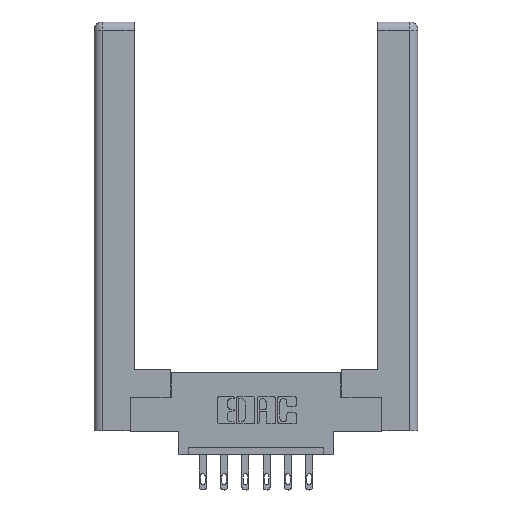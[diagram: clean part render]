
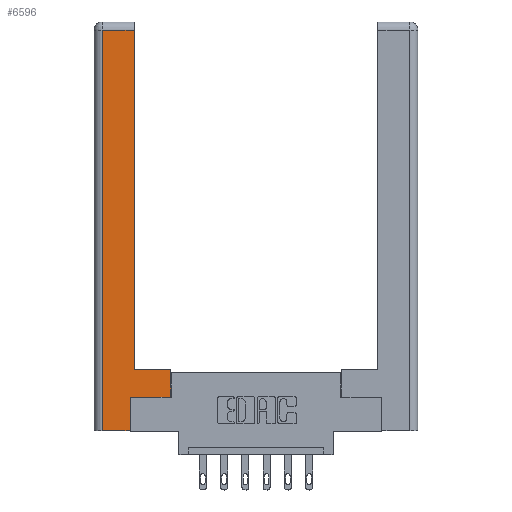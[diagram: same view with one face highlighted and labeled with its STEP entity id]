
A CAD part, top view. The second image highlights one B-rep face of the part: STEP entity #6596.
In plain terms, the highlighted planar face has unit normal (0, 0, 1).
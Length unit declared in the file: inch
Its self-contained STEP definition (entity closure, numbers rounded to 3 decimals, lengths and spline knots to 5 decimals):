
#57 = AXIS2_PLACEMENT_3D ( 'NONE', #5705, #9195, #6547 ) ;
#87 = CARTESIAN_POINT ( 'NONE',  ( 0.565, 0.45, 0. ) ) ;
#182 = LINE ( 'NONE', #9821, #8907 ) ;
#188 = DIRECTION ( 'NONE',  ( -1., 0., 0. ) ) ;
#192 = CARTESIAN_POINT ( 'NONE',  ( 0.0615, 0., 0. ) ) ;
#220 = DIRECTION ( 'NONE',  ( 0., 1., 0. ) ) ;
#345 = LINE ( 'NONE', #87, #2382 ) ;
#414 = FACE_OUTER_BOUND ( 'NONE', #2441, .T. ) ;
#625 = CARTESIAN_POINT ( 'NONE',  ( 0.295, 3., 0. ) ) ;
#692 = CARTESIAN_POINT ( 'NONE',  ( 0.0615, 2.94, 0. ) ) ;
#757 = CARTESIAN_POINT ( 'NONE',  ( 0.565, 0.45, 0. ) ) ;
#875 = LINE ( 'NONE', #4035, #4352 ) ;
#1170 = DIRECTION ( 'NONE',  ( 0., -1., 0. ) ) ;
#1419 = DIRECTION ( 'NONE',  ( 1., 0., 0. ) ) ;
#1443 = ORIENTED_EDGE ( 'NONE', *, *, #10647, .T. ) ;
#1577 = CARTESIAN_POINT ( 'NONE',  ( 0.265, 0., 0. ) ) ;
#1933 = ORIENTED_EDGE ( 'NONE', *, *, #9847, .T. ) ;
#2232 = VERTEX_POINT ( 'NONE', #1577 ) ;
#2312 = VERTEX_POINT ( 'NONE', #3712 ) ;
#2349 = CARTESIAN_POINT ( 'NONE',  ( 0.265, 0., 0. ) ) ;
#2382 = VECTOR ( 'NONE', #9279, 39.37008 ) ;
#2406 = ORIENTED_EDGE ( 'NONE', *, *, #5394, .T. ) ;
#2441 = EDGE_LOOP ( 'NONE', ( #3997, #5386, #6821, #2406, #8994, #1933, #6536, #1443 ) ) ;
#2784 = CARTESIAN_POINT ( 'NONE',  ( 0.0615, 0., 0. ) ) ;
#3058 = CARTESIAN_POINT ( 'NONE',  ( 0.295, 2.94, 0. ) ) ;
#3161 = EDGE_CURVE ( 'NONE', #2232, #4974, #3533, .T. ) ;
#3224 = VECTOR ( 'NONE', #9689, 39.37008 ) ;
#3470 = CARTESIAN_POINT ( 'NONE',  ( 0.565, 0.245, 0. ) ) ;
#3533 = LINE ( 'NONE', #6516, #9056 ) ;
#3712 = CARTESIAN_POINT ( 'NONE',  ( 0.295, 0.45, 0. ) ) ;
#3997 = ORIENTED_EDGE ( 'NONE', *, *, #7509, .T. ) ;
#4012 = EDGE_CURVE ( 'NONE', #9535, #5421, #4650, .T. ) ;
#4035 = CARTESIAN_POINT ( 'NONE',  ( 0.295, 0.45, 0. ) ) ;
#4266 = DIRECTION ( 'NONE',  ( 0., 1., 0. ) ) ;
#4352 = VECTOR ( 'NONE', #188, 39.37008 ) ;
#4417 = LINE ( 'NONE', #192, #9095 ) ;
#4650 = LINE ( 'NONE', #692, #3224 ) ;
#4974 = VERTEX_POINT ( 'NONE', #7138 ) ;
#5315 = DIRECTION ( 'NONE',  ( 1., 0., 0. ) ) ;
#5386 = ORIENTED_EDGE ( 'NONE', *, *, #4012, .T. ) ;
#5394 = EDGE_CURVE ( 'NONE', #10939, #2232, #9746, .T. ) ;
#5421 = VERTEX_POINT ( 'NONE', #10515 ) ;
#5469 = VECTOR ( 'NONE', #1419, 39.37008 ) ;
#5705 = CARTESIAN_POINT ( 'NONE',  ( 0., 0., 0. ) ) ;
#5869 = VERTEX_POINT ( 'NONE', #3470 ) ;
#6516 = CARTESIAN_POINT ( 'NONE',  ( 0.265, 0.245, 0. ) ) ;
#6536 = ORIENTED_EDGE ( 'NONE', *, *, #8911, .T. ) ;
#6547 = DIRECTION ( 'NONE',  ( -1., 0., 0. ) ) ;
#6596 = ADVANCED_FACE ( 'NONE', ( #414 ), #8288, .F. ) ;
#6821 = ORIENTED_EDGE ( 'NONE', *, *, #7190, .T. ) ;
#7138 = CARTESIAN_POINT ( 'NONE',  ( 0.265, 0.245, 0. ) ) ;
#7190 = EDGE_CURVE ( 'NONE', #5421, #10939, #4417, .T. ) ;
#7509 = EDGE_CURVE ( 'NONE', #2312, #9535, #8799, .T. ) ;
#7667 = VECTOR ( 'NONE', #4266, 39.37008 ) ;
#8288 = PLANE ( 'NONE',  #57 ) ;
#8776 = VERTEX_POINT ( 'NONE', #757 ) ;
#8799 = LINE ( 'NONE', #625, #7667 ) ;
#8907 = VECTOR ( 'NONE', #5315, 39.37008 ) ;
#8911 = EDGE_CURVE ( 'NONE', #5869, #8776, #345, .T. ) ;
#8994 = ORIENTED_EDGE ( 'NONE', *, *, #3161, .T. ) ;
#9056 = VECTOR ( 'NONE', #220, 39.37008 ) ;
#9095 = VECTOR ( 'NONE', #1170, 39.37008 ) ;
#9195 = DIRECTION ( 'NONE',  ( 0., 0., -1. ) ) ;
#9279 = DIRECTION ( 'NONE',  ( 0., 1., 0. ) ) ;
#9535 = VERTEX_POINT ( 'NONE', #3058 ) ;
#9689 = DIRECTION ( 'NONE',  ( -1., 0., 0. ) ) ;
#9746 = LINE ( 'NONE', #2349, #5469 ) ;
#9821 = CARTESIAN_POINT ( 'NONE',  ( 0.565, 0.245, 0. ) ) ;
#9847 = EDGE_CURVE ( 'NONE', #4974, #5869, #182, .T. ) ;
#10515 = CARTESIAN_POINT ( 'NONE',  ( 0.0615, 2.94, 0. ) ) ;
#10647 = EDGE_CURVE ( 'NONE', #8776, #2312, #875, .T. ) ;
#10939 = VERTEX_POINT ( 'NONE', #2784 ) ;
